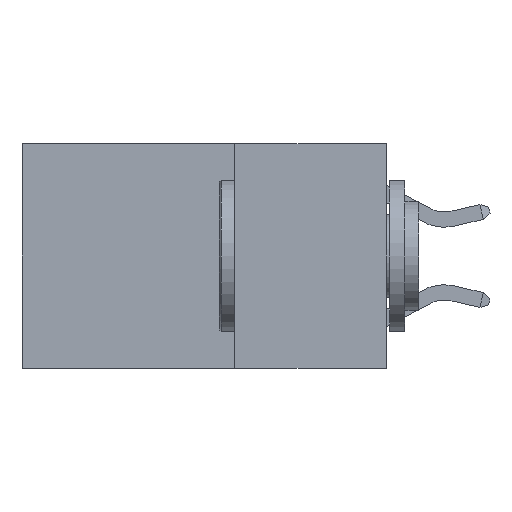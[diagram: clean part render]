
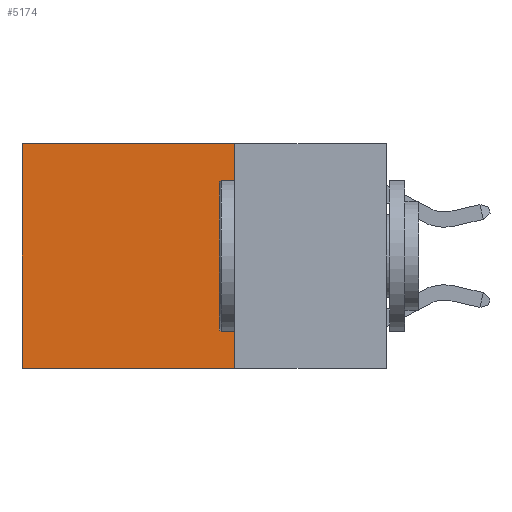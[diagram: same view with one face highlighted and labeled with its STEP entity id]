
A CAD part, left-side view. The second image highlights one B-rep face of the part: STEP entity #5174.
In plain terms, the highlighted planar face has unit normal (-1, 0, 0).
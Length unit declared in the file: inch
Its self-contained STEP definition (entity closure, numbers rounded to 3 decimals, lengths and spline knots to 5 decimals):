
#541 = PLANE ( 'NONE',  #2455 ) ;
#1451 = LINE ( 'NONE', #12469, #4044 ) ;
#2455 = AXIS2_PLACEMENT_3D ( 'NONE', #4530, #6602, #4621 ) ;
#3032 = LINE ( 'NONE', #11299, #10417 ) ;
#3959 = VERTEX_POINT ( 'NONE', #9508 ) ;
#3974 = CARTESIAN_POINT ( 'NONE',  ( 0.2625, 0.25, -0.37 ) ) ;
#4044 = VECTOR ( 'NONE', #9321, 39.37008 ) ;
#4074 = DIRECTION ( 'NONE',  ( 0., 1., 0. ) ) ;
#4251 = DIRECTION ( 'NONE',  ( 0., 1., 0. ) ) ;
#4465 = EDGE_CURVE ( 'NONE', #6925, #3959, #1451, .T. ) ;
#4530 = CARTESIAN_POINT ( 'NONE',  ( 0.2625, 0.25, 0. ) ) ;
#4621 = DIRECTION ( 'NONE',  ( 0., 0., -1. ) ) ;
#4698 = CARTESIAN_POINT ( 'NONE',  ( 0.2625, 0.25, 0. ) ) ;
#4765 = CARTESIAN_POINT ( 'NONE',  ( 0.2625, 0.6, -0.37 ) ) ;
#4856 = VECTOR ( 'NONE', #9472, 39.37008 ) ;
#5174 = ADVANCED_FACE ( 'NONE', ( #6610 ), #541, .F. ) ;
#5175 = LINE ( 'NONE', #8440, #4856 ) ;
#5336 = EDGE_CURVE ( 'NONE', #3959, #9857, #12817, .T. ) ;
#6231 = VERTEX_POINT ( 'NONE', #12765 ) ;
#6602 = DIRECTION ( 'NONE',  ( 1., 0., 0. ) ) ;
#6610 = FACE_OUTER_BOUND ( 'NONE', #9733, .T. ) ;
#6925 = VERTEX_POINT ( 'NONE', #4698 ) ;
#7082 = VECTOR ( 'NONE', #4251, 39.37008 ) ;
#7872 = ORIENTED_EDGE ( 'NONE', *, *, #5336, .F. ) ;
#8440 = CARTESIAN_POINT ( 'NONE',  ( 0.2625, 0.6, 0. ) ) ;
#9321 = DIRECTION ( 'NONE',  ( 0., 0., -1. ) ) ;
#9325 = EDGE_CURVE ( 'NONE', #6231, #9857, #5175, .T. ) ;
#9472 = DIRECTION ( 'NONE',  ( 0., 0., -1. ) ) ;
#9508 = CARTESIAN_POINT ( 'NONE',  ( 0.2625, 0.25, -0.37 ) ) ;
#9733 = EDGE_LOOP ( 'NONE', ( #10791, #7872, #12233, #12126 ) ) ;
#9857 = VERTEX_POINT ( 'NONE', #4765 ) ;
#10417 = VECTOR ( 'NONE', #4074, 39.37008 ) ;
#10791 = ORIENTED_EDGE ( 'NONE', *, *, #9325, .T. ) ;
#10900 = EDGE_CURVE ( 'NONE', #6925, #6231, #3032, .T. ) ;
#11299 = CARTESIAN_POINT ( 'NONE',  ( 0.2625, 0.25, 0. ) ) ;
#12126 = ORIENTED_EDGE ( 'NONE', *, *, #10900, .T. ) ;
#12233 = ORIENTED_EDGE ( 'NONE', *, *, #4465, .F. ) ;
#12469 = CARTESIAN_POINT ( 'NONE',  ( 0.2625, 0.25, 0. ) ) ;
#12765 = CARTESIAN_POINT ( 'NONE',  ( 0.2625, 0.6, 0. ) ) ;
#12817 = LINE ( 'NONE', #3974, #7082 ) ;
